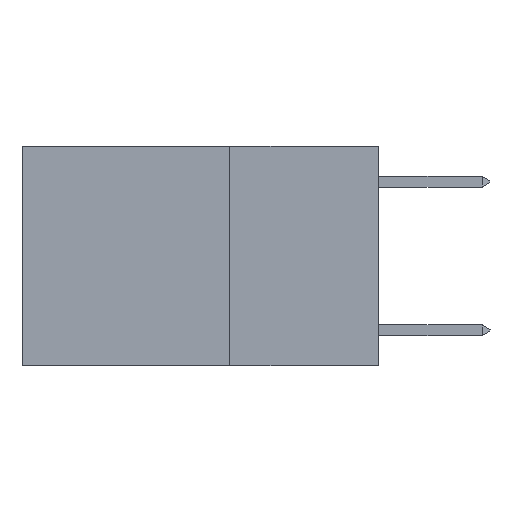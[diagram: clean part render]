
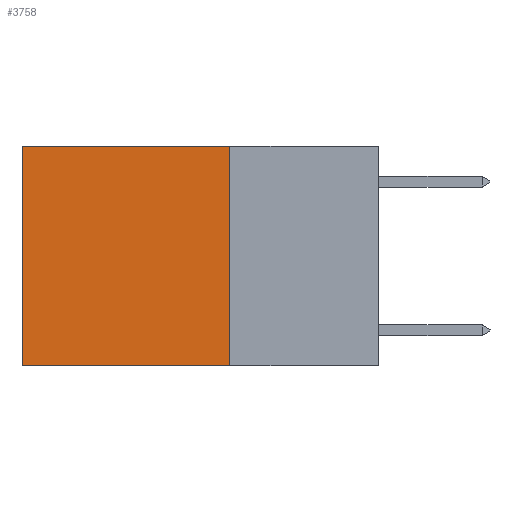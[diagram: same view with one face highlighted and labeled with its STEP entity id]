
A CAD part, left-side view. The second image highlights one B-rep face of the part: STEP entity #3758.
In plain terms, the highlighted planar face has unit normal (-1, 0, 0).
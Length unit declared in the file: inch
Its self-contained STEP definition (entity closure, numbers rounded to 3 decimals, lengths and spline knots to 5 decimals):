
#175 = ORIENTED_EDGE ( 'NONE', *, *, #18840, .F. ) ;
#284 = VERTEX_POINT ( 'NONE', #3355 ) ;
#2124 = VERTEX_POINT ( 'NONE', #7696 ) ;
#2583 = EDGE_CURVE ( 'NONE', #15091, #2124, #10631, .T. ) ;
#3355 = CARTESIAN_POINT ( 'NONE',  ( 0.2625, 0.6, 0. ) ) ;
#3758 = ADVANCED_FACE ( 'NONE', ( #26372 ), #22950, .F. ) ;
#6238 = DIRECTION ( 'NONE',  ( 0., 0., -1. ) ) ;
#6254 = CARTESIAN_POINT ( 'NONE',  ( 0.2625, 0.25, 0. ) ) ;
#7297 = DIRECTION ( 'NONE',  ( 0., 1., 0. ) ) ;
#7696 = CARTESIAN_POINT ( 'NONE',  ( 0.2625, 0.6, -0.37 ) ) ;
#7911 = CARTESIAN_POINT ( 'NONE',  ( 0.2625, 0.25, 0. ) ) ;
#10534 = CARTESIAN_POINT ( 'NONE',  ( 0.2625, 0.6, 0. ) ) ;
#10631 = LINE ( 'NONE', #11055, #14211 ) ;
#11055 = CARTESIAN_POINT ( 'NONE',  ( 0.2625, 0.25, -0.37 ) ) ;
#11160 = ORIENTED_EDGE ( 'NONE', *, *, #12519, .T. ) ;
#11296 = DIRECTION ( 'NONE',  ( 0., 1., 0. ) ) ;
#11436 = CARTESIAN_POINT ( 'NONE',  ( 0.2625, 0.25, 0. ) ) ;
#12519 = EDGE_CURVE ( 'NONE', #25912, #284, #15858, .T. ) ;
#14169 = CARTESIAN_POINT ( 'NONE',  ( 0.2625, 0.25, -0.37 ) ) ;
#14211 = VECTOR ( 'NONE', #11296, 39.37008 ) ;
#14356 = VECTOR ( 'NONE', #7297, 39.37008 ) ;
#15091 = VERTEX_POINT ( 'NONE', #14169 ) ;
#15858 = LINE ( 'NONE', #7911, #14356 ) ;
#17005 = VECTOR ( 'NONE', #29067, 39.37008 ) ;
#17736 = LINE ( 'NONE', #10534, #17005 ) ;
#18237 = VECTOR ( 'NONE', #6238, 39.37008 ) ;
#18302 = LINE ( 'NONE', #11436, #18237 ) ;
#18840 = EDGE_CURVE ( 'NONE', #25912, #15091, #18302, .T. ) ;
#19659 = AXIS2_PLACEMENT_3D ( 'NONE', #22977, #23309, #22879 ) ;
#22879 = DIRECTION ( 'NONE',  ( 0., 0., -1. ) ) ;
#22950 = PLANE ( 'NONE',  #19659 ) ;
#22977 = CARTESIAN_POINT ( 'NONE',  ( 0.2625, 0.25, 0. ) ) ;
#22997 = ORIENTED_EDGE ( 'NONE', *, *, #2583, .F. ) ;
#23309 = DIRECTION ( 'NONE',  ( 1., 0., 0. ) ) ;
#24738 = EDGE_LOOP ( 'NONE', ( #25027, #22997, #175, #11160 ) ) ;
#25027 = ORIENTED_EDGE ( 'NONE', *, *, #27120, .T. ) ;
#25912 = VERTEX_POINT ( 'NONE', #6254 ) ;
#26372 = FACE_OUTER_BOUND ( 'NONE', #24738, .T. ) ;
#27120 = EDGE_CURVE ( 'NONE', #284, #2124, #17736, .T. ) ;
#29067 = DIRECTION ( 'NONE',  ( 0., 0., -1. ) ) ;
